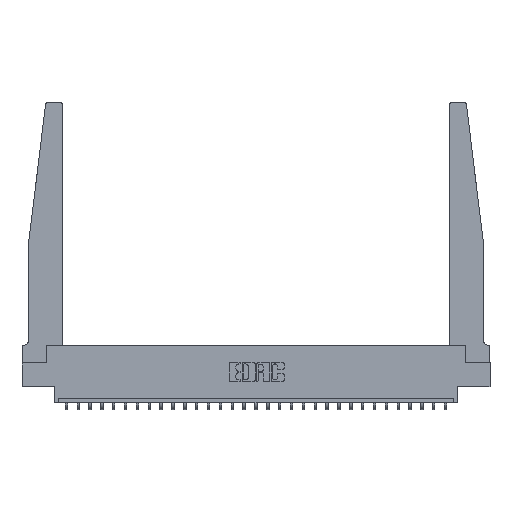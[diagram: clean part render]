
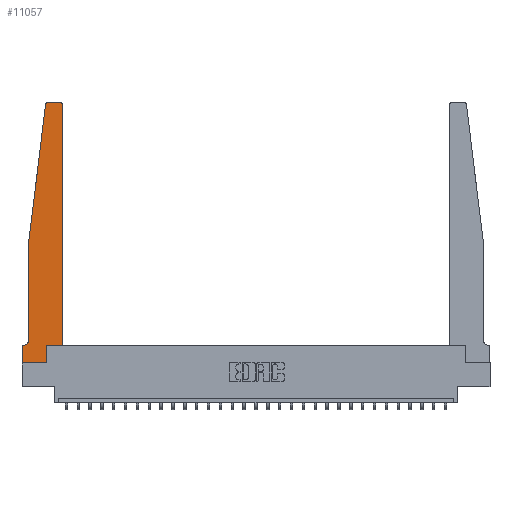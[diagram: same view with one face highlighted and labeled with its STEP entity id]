
A CAD part, top view. The second image highlights one B-rep face of the part: STEP entity #11057.
In plain terms, the highlighted planar face has unit normal (0, 0, 1).
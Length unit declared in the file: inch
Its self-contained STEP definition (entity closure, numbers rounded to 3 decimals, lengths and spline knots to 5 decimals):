
#30 = CARTESIAN_POINT ( 'NONE',  ( 0.27653, 2.75, 0.37 ) ) ;
#191 = VERTEX_POINT ( 'NONE', #12546 ) ;
#604 = DIRECTION ( 'NONE',  ( 0., -1., 0. ) ) ;
#625 = VECTOR ( 'NONE', #668, 39.37008 ) ;
#643 = EDGE_CURVE ( 'NONE', #4840, #22242, #24693, .T. ) ;
#668 = DIRECTION ( 'NONE',  ( -0.122, -0.992, 0. ) ) ;
#956 = VERTEX_POINT ( 'NONE', #25526 ) ;
#1384 = VERTEX_POINT ( 'NONE', #30 ) ;
#1604 = VERTEX_POINT ( 'NONE', #17330 ) ;
#2034 = ORIENTED_EDGE ( 'NONE', *, *, #22602, .T. ) ;
#3033 = VERTEX_POINT ( 'NONE', #26087 ) ;
#3180 = CARTESIAN_POINT ( 'NONE',  ( 0.425, 0.18, 0.37 ) ) ;
#3523 = EDGE_LOOP ( 'NONE', ( #23672, #21996, #2034, #7399, #18749, #25979, #10472, #10908, #23691, #9285, #5526, #11294 ) ) ;
#3614 = PLANE ( 'NONE',  #15678 ) ;
#3660 = AXIS2_PLACEMENT_3D ( 'NONE', #22501, #10225, #24579 ) ;
#3826 = VERTEX_POINT ( 'NONE', #10040 ) ;
#4184 = CARTESIAN_POINT ( 'NONE',  ( 0.2605, 0., 0.37 ) ) ;
#4840 = VERTEX_POINT ( 'NONE', #24390 ) ;
#4986 = EDGE_CURVE ( 'NONE', #22242, #956, #10699, .T. ) ;
#5002 = VECTOR ( 'NONE', #12826, 39.37008 ) ;
#5526 = ORIENTED_EDGE ( 'NONE', *, *, #4986, .T. ) ;
#5653 = LINE ( 'NONE', #25118, #5002 ) ;
#5720 = EDGE_CURVE ( 'NONE', #6719, #1384, #22055, .T. ) ;
#5752 = CARTESIAN_POINT ( 'NONE',  ( 0., 0., 0.37 ) ) ;
#5768 = VECTOR ( 'NONE', #14019, 39.37008 ) ;
#6594 = EDGE_CURVE ( 'NONE', #15794, #4840, #18463, .T. ) ;
#6651 = CIRCLE ( 'NONE', #22726, 0.05 ) ;
#6661 = FACE_OUTER_BOUND ( 'NONE', #3523, .T. ) ;
#6719 = VERTEX_POINT ( 'NONE', #16479 ) ;
#7399 = ORIENTED_EDGE ( 'NONE', *, *, #18384, .T. ) ;
#7733 = DIRECTION ( 'NONE',  ( 0., 0., 1. ) ) ;
#8890 = CARTESIAN_POINT ( 'NONE',  ( 0., 0., 0.37 ) ) ;
#8916 = CARTESIAN_POINT ( 'NONE',  ( 0.065, 1.25, 0.37 ) ) ;
#9285 = ORIENTED_EDGE ( 'NONE', *, *, #643, .T. ) ;
#9300 = DIRECTION ( 'NONE',  ( 0., 0., -1. ) ) ;
#9356 = LINE ( 'NONE', #9883, #24441 ) ;
#9876 = CIRCLE ( 'NONE', #3660, 0.03 ) ;
#9883 = CARTESIAN_POINT ( 'NONE',  ( 0., 0., 0.37 ) ) ;
#10040 = CARTESIAN_POINT ( 'NONE',  ( 0.015, 0.1875, 0.37 ) ) ;
#10225 = DIRECTION ( 'NONE',  ( 0., 0., 1. ) ) ;
#10334 = CARTESIAN_POINT ( 'NONE',  ( 0.065, 1.25, 0.37 ) ) ;
#10472 = ORIENTED_EDGE ( 'NONE', *, *, #16563, .T. ) ;
#10574 = LINE ( 'NONE', #10334, #20841 ) ;
#10657 = CARTESIAN_POINT ( 'NONE',  ( 0.425, 0.18, 0.37 ) ) ;
#10699 = LINE ( 'NONE', #10657, #26422 ) ;
#10908 = ORIENTED_EDGE ( 'NONE', *, *, #15072, .T. ) ;
#11057 = ADVANCED_FACE ( 'NONE', ( #6661 ), #3614, .T. ) ;
#11250 = CARTESIAN_POINT ( 'NONE',  ( 0.25, 2.75, 0.37 ) ) ;
#11294 = ORIENTED_EDGE ( 'NONE', *, *, #11668, .T. ) ;
#11346 = VERTEX_POINT ( 'NONE', #8890 ) ;
#11668 = EDGE_CURVE ( 'NONE', #956, #6719, #9876, .T. ) ;
#11892 = LINE ( 'NONE', #5752, #5768 ) ;
#11957 = DIRECTION ( 'NONE',  ( 0., 0., 1. ) ) ;
#12546 = CARTESIAN_POINT ( 'NONE',  ( 0.065, 1.25, 0.37 ) ) ;
#12826 = DIRECTION ( 'NONE',  ( -1., 0., 0. ) ) ;
#13027 = VECTOR ( 'NONE', #16042, 39.37008 ) ;
#13786 = VECTOR ( 'NONE', #24574, 39.37008 ) ;
#14019 = DIRECTION ( 'NONE',  ( 0., -1., 0. ) ) ;
#14051 = VERTEX_POINT ( 'NONE', #14478 ) ;
#14478 = CARTESIAN_POINT ( 'NONE',  ( 0.24675, 2.72367, 0.37 ) ) ;
#15072 = EDGE_CURVE ( 'NONE', #11346, #15794, #9356, .T. ) ;
#15678 = AXIS2_PLACEMENT_3D ( 'NONE', #20051, #7733, #22098 ) ;
#15794 = VERTEX_POINT ( 'NONE', #4184 ) ;
#16042 = DIRECTION ( 'NONE',  ( 0., 1., 0. ) ) ;
#16260 = CIRCLE ( 'NONE', #23028, 0.03 ) ;
#16307 = CARTESIAN_POINT ( 'NONE',  ( 0.425, 0.18, 0.37 ) ) ;
#16479 = CARTESIAN_POINT ( 'NONE',  ( 0.395, 2.75, 0.37 ) ) ;
#16563 = EDGE_CURVE ( 'NONE', #3033, #11346, #11892, .T. ) ;
#16577 = VECTOR ( 'NONE', #25693, 39.37008 ) ;
#17066 = LINE ( 'NONE', #8916, #625 ) ;
#17330 = CARTESIAN_POINT ( 'NONE',  ( 0.065, 0.2375, 0.37 ) ) ;
#18384 = EDGE_CURVE ( 'NONE', #191, #1604, #10574, .T. ) ;
#18463 = LINE ( 'NONE', #26284, #13027 ) ;
#18749 = ORIENTED_EDGE ( 'NONE', *, *, #25214, .T. ) ;
#18889 = DIRECTION ( 'NONE',  ( 0., 1., 0. ) ) ;
#20036 = EDGE_CURVE ( 'NONE', #1384, #14051, #16260, .T. ) ;
#20051 = CARTESIAN_POINT ( 'NONE',  ( 0., 0.1875, 0.37 ) ) ;
#20281 = EDGE_CURVE ( 'NONE', #3826, #3033, #5653, .T. ) ;
#20841 = VECTOR ( 'NONE', #604, 39.37008 ) ;
#21585 = CARTESIAN_POINT ( 'NONE',  ( 0.015, 0.2375, 0.37 ) ) ;
#21996 = ORIENTED_EDGE ( 'NONE', *, *, #20036, .T. ) ;
#22055 = LINE ( 'NONE', #11250, #16577 ) ;
#22098 = DIRECTION ( 'NONE',  ( 1., 0., 0. ) ) ;
#22168 = DIRECTION ( 'NONE',  ( 1., 0., 0. ) ) ;
#22242 = VERTEX_POINT ( 'NONE', #3180 ) ;
#22501 = CARTESIAN_POINT ( 'NONE',  ( 0.395, 2.72, 0.37 ) ) ;
#22602 = EDGE_CURVE ( 'NONE', #14051, #191, #17066, .T. ) ;
#22726 = AXIS2_PLACEMENT_3D ( 'NONE', #21585, #9300, #23662 ) ;
#23028 = AXIS2_PLACEMENT_3D ( 'NONE', #24246, #11957, #26309 ) ;
#23662 = DIRECTION ( 'NONE',  ( -1., 0., 0. ) ) ;
#23672 = ORIENTED_EDGE ( 'NONE', *, *, #5720, .T. ) ;
#23691 = ORIENTED_EDGE ( 'NONE', *, *, #6594, .T. ) ;
#24246 = CARTESIAN_POINT ( 'NONE',  ( 0.27653, 2.72, 0.37 ) ) ;
#24390 = CARTESIAN_POINT ( 'NONE',  ( 0.2605, 0.18, 0.37 ) ) ;
#24441 = VECTOR ( 'NONE', #22168, 39.37008 ) ;
#24574 = DIRECTION ( 'NONE',  ( 1., 0., 0. ) ) ;
#24579 = DIRECTION ( 'NONE',  ( 1., 0., 0. ) ) ;
#24693 = LINE ( 'NONE', #16307, #13786 ) ;
#25118 = CARTESIAN_POINT ( 'NONE',  ( 0.065, 0.1875, 0.37 ) ) ;
#25214 = EDGE_CURVE ( 'NONE', #1604, #3826, #6651, .T. ) ;
#25526 = CARTESIAN_POINT ( 'NONE',  ( 0.425, 2.72, 0.37 ) ) ;
#25693 = DIRECTION ( 'NONE',  ( -1., 0., 0. ) ) ;
#25979 = ORIENTED_EDGE ( 'NONE', *, *, #20281, .T. ) ;
#26087 = CARTESIAN_POINT ( 'NONE',  ( 0., 0.1875, 0.37 ) ) ;
#26284 = CARTESIAN_POINT ( 'NONE',  ( 0.2605, 0.18, 0.37 ) ) ;
#26309 = DIRECTION ( 'NONE',  ( 1., 0., 0. ) ) ;
#26422 = VECTOR ( 'NONE', #18889, 39.37008 ) ;
